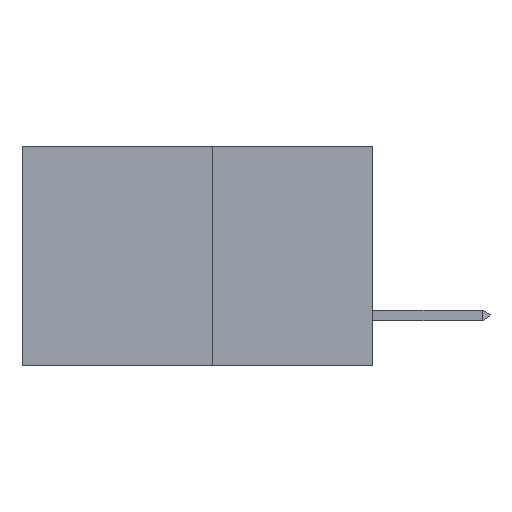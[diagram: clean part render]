
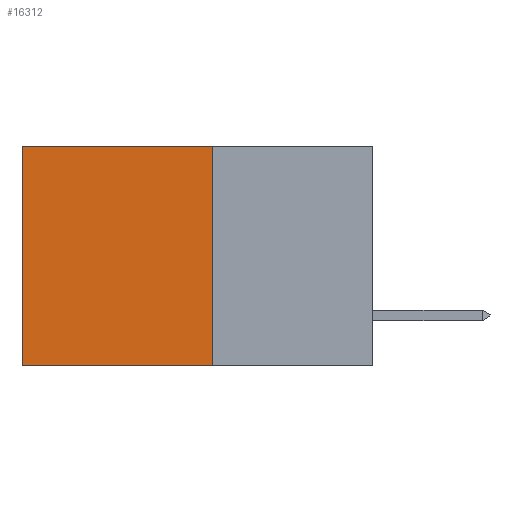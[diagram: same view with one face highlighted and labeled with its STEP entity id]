
A CAD part, left-side view. The second image highlights one B-rep face of the part: STEP entity #16312.
In plain terms, the highlighted planar face has unit normal (-1, 0, 0).
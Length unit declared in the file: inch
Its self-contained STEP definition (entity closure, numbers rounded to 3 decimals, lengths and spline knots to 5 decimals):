
#166 = CARTESIAN_POINT ( 'NONE',  ( 0.277, 0.59, 0. ) ) ;
#221 = LINE ( 'NONE', #15019, #12245 ) ;
#421 = DIRECTION ( 'NONE',  ( 1., 0., 0. ) ) ;
#773 = VECTOR ( 'NONE', #18074, 39.37008 ) ;
#962 = ORIENTED_EDGE ( 'NONE', *, *, #3262, .F. ) ;
#1190 = CARTESIAN_POINT ( 'NONE',  ( 0.277, 0.27, -0.37 ) ) ;
#1404 = DIRECTION ( 'NONE',  ( 0., 1., 0. ) ) ;
#2106 = VERTEX_POINT ( 'NONE', #12415 ) ;
#3262 = EDGE_CURVE ( 'NONE', #5827, #2106, #6475, .T. ) ;
#3771 = VECTOR ( 'NONE', #12159, 39.37008 ) ;
#4075 = VERTEX_POINT ( 'NONE', #7867 ) ;
#5484 = LINE ( 'NONE', #10802, #9585 ) ;
#5795 = DIRECTION ( 'NONE',  ( 0., 0., -1. ) ) ;
#5827 = VERTEX_POINT ( 'NONE', #13284 ) ;
#6168 = AXIS2_PLACEMENT_3D ( 'NONE', #9819, #421, #11382 ) ;
#6475 = LINE ( 'NONE', #19528, #773 ) ;
#7252 = ORIENTED_EDGE ( 'NONE', *, *, #11327, .T. ) ;
#7621 = EDGE_LOOP ( 'NONE', ( #7252, #962, #15380, #14144 ) ) ;
#7867 = CARTESIAN_POINT ( 'NONE',  ( 0.277, 0.27, 0. ) ) ;
#9585 = VECTOR ( 'NONE', #1404, 39.37008 ) ;
#9819 = CARTESIAN_POINT ( 'NONE',  ( 0.277, 0.27, -0.37 ) ) ;
#10802 = CARTESIAN_POINT ( 'NONE',  ( 0.277, 0.27, 0. ) ) ;
#11327 = EDGE_CURVE ( 'NONE', #17270, #2106, #221, .T. ) ;
#11382 = DIRECTION ( 'NONE',  ( 0., 0., -1. ) ) ;
#11403 = EDGE_CURVE ( 'NONE', #4075, #5827, #15188, .T. ) ;
#11493 = EDGE_CURVE ( 'NONE', #4075, #17270, #5484, .T. ) ;
#12159 = DIRECTION ( 'NONE',  ( 0., 0., -1. ) ) ;
#12245 = VECTOR ( 'NONE', #5795, 39.37008 ) ;
#12415 = CARTESIAN_POINT ( 'NONE',  ( 0.277, 0.59, -0.37 ) ) ;
#13284 = CARTESIAN_POINT ( 'NONE',  ( 0.277, 0.27, -0.37 ) ) ;
#14144 = ORIENTED_EDGE ( 'NONE', *, *, #11493, .T. ) ;
#15019 = CARTESIAN_POINT ( 'NONE',  ( 0.277, 0.59, -0.37 ) ) ;
#15188 = LINE ( 'NONE', #1190, #3771 ) ;
#15380 = ORIENTED_EDGE ( 'NONE', *, *, #11403, .F. ) ;
#16312 = ADVANCED_FACE ( 'NONE', ( #19886 ), #17526, .F. ) ;
#17270 = VERTEX_POINT ( 'NONE', #166 ) ;
#17526 = PLANE ( 'NONE',  #6168 ) ;
#18074 = DIRECTION ( 'NONE',  ( 0., 1., 0. ) ) ;
#19528 = CARTESIAN_POINT ( 'NONE',  ( 0.277, 0.27, -0.37 ) ) ;
#19886 = FACE_OUTER_BOUND ( 'NONE', #7621, .T. ) ;
